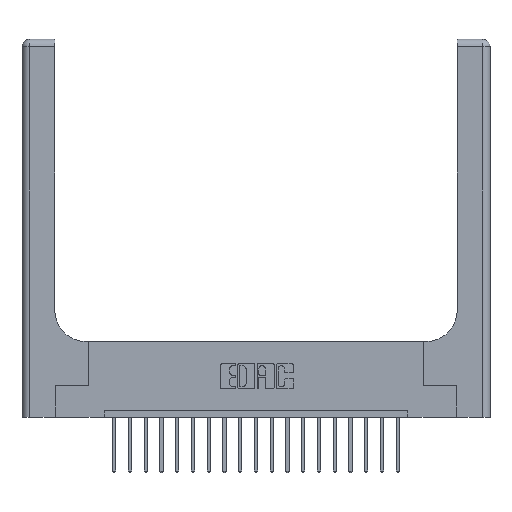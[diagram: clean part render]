
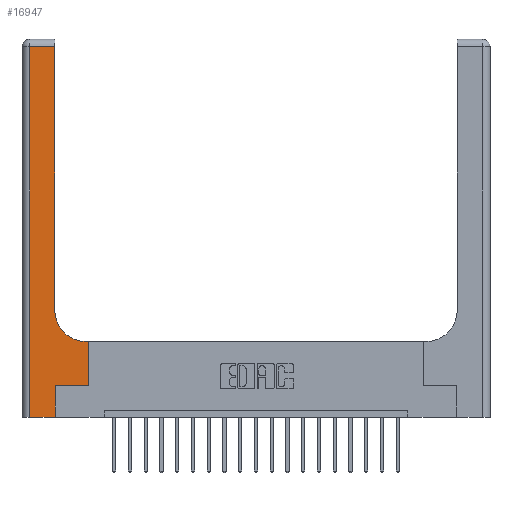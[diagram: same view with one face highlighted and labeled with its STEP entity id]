
A CAD part, top view. The second image highlights one B-rep face of the part: STEP entity #16947.
In plain terms, the highlighted planar face has unit normal (0, 0, 1).
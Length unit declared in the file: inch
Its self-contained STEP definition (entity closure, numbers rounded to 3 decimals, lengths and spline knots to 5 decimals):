
#205 = VERTEX_POINT ( 'NONE', #19949 ) ;
#435 = VECTOR ( 'NONE', #10525, 39.37008 ) ;
#582 = VECTOR ( 'NONE', #7415, 39.37008 ) ;
#626 = VECTOR ( 'NONE', #20391, 39.37008 ) ;
#1599 = DIRECTION ( 'NONE',  ( -1., 0., 0. ) ) ;
#1605 = VECTOR ( 'NONE', #1599, 39.37008 ) ;
#1943 = CARTESIAN_POINT ( 'NONE',  ( 0., 2.94, 0.37 ) ) ;
#2414 = VERTEX_POINT ( 'NONE', #10575 ) ;
#2555 = VERTEX_POINT ( 'NONE', #10992 ) ;
#2899 = ORIENTED_EDGE ( 'NONE', *, *, #20038, .T. ) ;
#2941 = CARTESIAN_POINT ( 'NONE',  ( 0.265, 0.25, 0.37 ) ) ;
#3115 = CARTESIAN_POINT ( 'NONE',  ( 0.26, 0.85, 0.37 ) ) ;
#3289 = VERTEX_POINT ( 'NONE', #18530 ) ;
#3844 = FACE_OUTER_BOUND ( 'NONE', #11642, .T. ) ;
#4063 = ORIENTED_EDGE ( 'NONE', *, *, #11825, .T. ) ;
#4239 = CARTESIAN_POINT ( 'NONE',  ( 0.06, 0., 0.37 ) ) ;
#4298 = LINE ( 'NONE', #2941, #435 ) ;
#4862 = CARTESIAN_POINT ( 'NONE',  ( 0.528, 0.25, 0.37 ) ) ;
#5085 = DIRECTION ( 'NONE',  ( -1., 0., 0. ) ) ;
#5538 = EDGE_CURVE ( 'NONE', #9005, #9641, #9694, .T. ) ;
#5550 = CARTESIAN_POINT ( 'NONE',  ( 0.26, 3., 0.37 ) ) ;
#5750 = VECTOR ( 'NONE', #9607, 39.37008 ) ;
#6448 = VERTEX_POINT ( 'NONE', #4239 ) ;
#6462 = EDGE_CURVE ( 'NONE', #8674, #2555, #10884, .T. ) ;
#7415 = DIRECTION ( 'NONE',  ( 0., 1., 0. ) ) ;
#7920 = VERTEX_POINT ( 'NONE', #15843 ) ;
#8033 = ORIENTED_EDGE ( 'NONE', *, *, #20223, .T. ) ;
#8281 = DIRECTION ( 'NONE',  ( -1., 0., 0. ) ) ;
#8481 = VECTOR ( 'NONE', #9507, 39.37008 ) ;
#8487 = CARTESIAN_POINT ( 'NONE',  ( 0., 3., 0.37 ) ) ;
#8674 = VERTEX_POINT ( 'NONE', #8845 ) ;
#8845 = CARTESIAN_POINT ( 'NONE',  ( 0.528, 0.25, 0.37 ) ) ;
#9005 = VERTEX_POINT ( 'NONE', #3115 ) ;
#9373 = ORIENTED_EDGE ( 'NONE', *, *, #19354, .T. ) ;
#9507 = DIRECTION ( 'NONE',  ( 0., 1., 0. ) ) ;
#9536 = LINE ( 'NONE', #1943, #15211 ) ;
#9607 = DIRECTION ( 'NONE',  ( 0., 1., 0. ) ) ;
#9641 = VERTEX_POINT ( 'NONE', #17681 ) ;
#9694 = LINE ( 'NONE', #5550, #582 ) ;
#9705 = VECTOR ( 'NONE', #14935, 39.37008 ) ;
#9857 = EDGE_CURVE ( 'NONE', #7920, #8674, #4298, .T. ) ;
#10525 = DIRECTION ( 'NONE',  ( 1., 0., 0. ) ) ;
#10575 = CARTESIAN_POINT ( 'NONE',  ( 0.265, 0., 0.37 ) ) ;
#10690 = DIRECTION ( 'NONE',  ( 1., 0., 0. ) ) ;
#10827 = LINE ( 'NONE', #18624, #626 ) ;
#10884 = LINE ( 'NONE', #4862, #5750 ) ;
#10992 = CARTESIAN_POINT ( 'NONE',  ( 0.528, 0.6, 0.37 ) ) ;
#11077 = LINE ( 'NONE', #17407, #8481 ) ;
#11168 = AXIS2_PLACEMENT_3D ( 'NONE', #8487, #13194, #5085 ) ;
#11642 = EDGE_LOOP ( 'NONE', ( #12185, #8033, #19615, #4063, #15200, #14430, #15659, #9373, #2899 ) ) ;
#11825 = EDGE_CURVE ( 'NONE', #6448, #2414, #13513, .T. ) ;
#12185 = ORIENTED_EDGE ( 'NONE', *, *, #5538, .T. ) ;
#12524 = LINE ( 'NONE', #15808, #1605 ) ;
#13194 = DIRECTION ( 'NONE',  ( 0., 0., -1. ) ) ;
#13513 = LINE ( 'NONE', #19847, #9705 ) ;
#13919 = DIRECTION ( 'NONE',  ( 0., 0., -1. ) ) ;
#14234 = CARTESIAN_POINT ( 'NONE',  ( 0.51, 0.85, 0.37 ) ) ;
#14430 = ORIENTED_EDGE ( 'NONE', *, *, #9857, .T. ) ;
#14935 = DIRECTION ( 'NONE',  ( 1., 0., 0. ) ) ;
#15200 = ORIENTED_EDGE ( 'NONE', *, *, #16405, .T. ) ;
#15202 = CIRCLE ( 'NONE', #17856, 0.25 ) ;
#15211 = VECTOR ( 'NONE', #8281, 39.37008 ) ;
#15659 = ORIENTED_EDGE ( 'NONE', *, *, #6462, .T. ) ;
#15808 = CARTESIAN_POINT ( 'NONE',  ( 0.26, 0.6, 0.37 ) ) ;
#15843 = CARTESIAN_POINT ( 'NONE',  ( 0.265, 0.25, 0.37 ) ) ;
#16405 = EDGE_CURVE ( 'NONE', #2414, #7920, #11077, .T. ) ;
#16947 = ADVANCED_FACE ( 'NONE', ( #3844 ), #19631, .F. ) ;
#17407 = CARTESIAN_POINT ( 'NONE',  ( 0.265, 0., 0.37 ) ) ;
#17681 = CARTESIAN_POINT ( 'NONE',  ( 0.26, 2.94, 0.37 ) ) ;
#17856 = AXIS2_PLACEMENT_3D ( 'NONE', #14234, #13919, #10690 ) ;
#18530 = CARTESIAN_POINT ( 'NONE',  ( 0.51, 0.6, 0.37 ) ) ;
#18624 = CARTESIAN_POINT ( 'NONE',  ( 0.06, 3., 0.37 ) ) ;
#19354 = EDGE_CURVE ( 'NONE', #2555, #3289, #12524, .T. ) ;
#19615 = ORIENTED_EDGE ( 'NONE', *, *, #19652, .T. ) ;
#19631 = PLANE ( 'NONE',  #11168 ) ;
#19652 = EDGE_CURVE ( 'NONE', #205, #6448, #10827, .T. ) ;
#19847 = CARTESIAN_POINT ( 'NONE',  ( 0., 0., 0.37 ) ) ;
#19949 = CARTESIAN_POINT ( 'NONE',  ( 0.06, 2.94, 0.37 ) ) ;
#20038 = EDGE_CURVE ( 'NONE', #3289, #9005, #15202, .T. ) ;
#20223 = EDGE_CURVE ( 'NONE', #9641, #205, #9536, .T. ) ;
#20391 = DIRECTION ( 'NONE',  ( 0., -1., 0. ) ) ;
